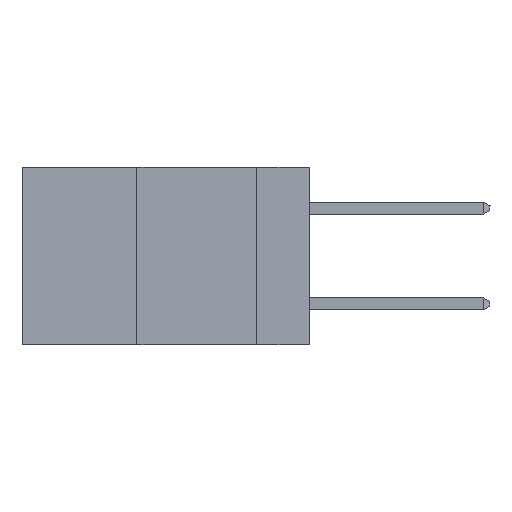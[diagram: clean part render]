
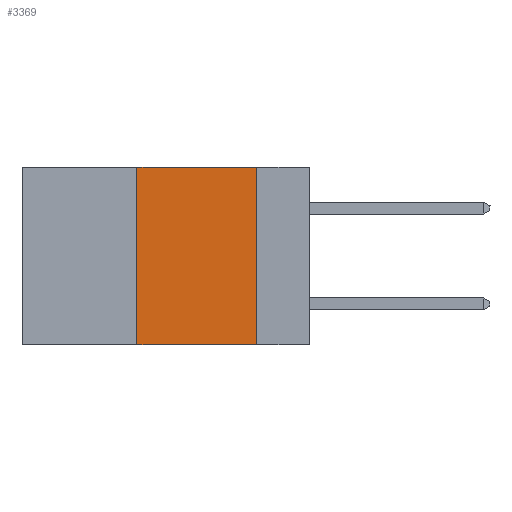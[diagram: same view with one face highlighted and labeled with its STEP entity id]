
A CAD part, left-side view. The second image highlights one B-rep face of the part: STEP entity #3369.
In plain terms, the highlighted planar face has unit normal (-1, 0, 0).
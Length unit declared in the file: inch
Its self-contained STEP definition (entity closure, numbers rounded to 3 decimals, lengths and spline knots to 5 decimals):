
#399 = DIRECTION ( 'NONE',  ( 1., 0., 0. ) ) ;
#416 = CARTESIAN_POINT ( 'NONE',  ( 0., 0.6, 0. ) ) ;
#962 = CARTESIAN_POINT ( 'NONE',  ( 0., 0.36, -0.37 ) ) ;
#1530 = EDGE_CURVE ( 'NONE', #1717, #6868, #10003, .T. ) ;
#1703 = CARTESIAN_POINT ( 'NONE',  ( 0., 0.11, 0. ) ) ;
#1717 = VERTEX_POINT ( 'NONE', #962 ) ;
#1822 = ORIENTED_EDGE ( 'NONE', *, *, #1530, .F. ) ;
#1831 = VECTOR ( 'NONE', #6701, 39.37008 ) ;
#2154 = CARTESIAN_POINT ( 'NONE',  ( 0., 0.11, -0.37 ) ) ;
#2412 = CARTESIAN_POINT ( 'NONE',  ( 0., 0.36, 0. ) ) ;
#2848 = EDGE_CURVE ( 'NONE', #11248, #9638, #9008, .T. ) ;
#3181 = ORIENTED_EDGE ( 'NONE', *, *, #7927, .T. ) ;
#3284 = EDGE_CURVE ( 'NONE', #6868, #11248, #11383, .T. ) ;
#3369 = ADVANCED_FACE ( 'NONE', ( #6994 ), #4842, .F. ) ;
#4576 = ORIENTED_EDGE ( 'NONE', *, *, #3284, .F. ) ;
#4842 = PLANE ( 'NONE',  #10904 ) ;
#4992 = CARTESIAN_POINT ( 'NONE',  ( 0., 0.36, 0. ) ) ;
#5177 = VECTOR ( 'NONE', #10300, 39.37008 ) ;
#5292 = DIRECTION ( 'NONE',  ( 0., 0., -1. ) ) ;
#6701 = DIRECTION ( 'NONE',  ( 0., -1., 0. ) ) ;
#6791 = EDGE_LOOP ( 'NONE', ( #8017, #4576, #1822, #3181 ) ) ;
#6868 = VERTEX_POINT ( 'NONE', #4992 ) ;
#6994 = FACE_OUTER_BOUND ( 'NONE', #6791, .T. ) ;
#7015 = VECTOR ( 'NONE', #8865, 39.37008 ) ;
#7026 = LINE ( 'NONE', #10201, #1831 ) ;
#7927 = EDGE_CURVE ( 'NONE', #1717, #9638, #7026, .T. ) ;
#8017 = ORIENTED_EDGE ( 'NONE', *, *, #2848, .F. ) ;
#8545 = DIRECTION ( 'NONE',  ( 0., -1., 0. ) ) ;
#8856 = VECTOR ( 'NONE', #8545, 39.37008 ) ;
#8865 = DIRECTION ( 'NONE',  ( 0., 0., -1. ) ) ;
#9008 = LINE ( 'NONE', #1703, #7015 ) ;
#9047 = CARTESIAN_POINT ( 'NONE',  ( 0., 0.6, 0. ) ) ;
#9638 = VERTEX_POINT ( 'NONE', #2154 ) ;
#10003 = LINE ( 'NONE', #2412, #5177 ) ;
#10201 = CARTESIAN_POINT ( 'NONE',  ( 0., 0.6, -0.37 ) ) ;
#10300 = DIRECTION ( 'NONE',  ( 0., 0., 1. ) ) ;
#10304 = CARTESIAN_POINT ( 'NONE',  ( 0., 0.11, 0. ) ) ;
#10904 = AXIS2_PLACEMENT_3D ( 'NONE', #9047, #399, #5292 ) ;
#11248 = VERTEX_POINT ( 'NONE', #10304 ) ;
#11383 = LINE ( 'NONE', #416, #8856 ) ;
